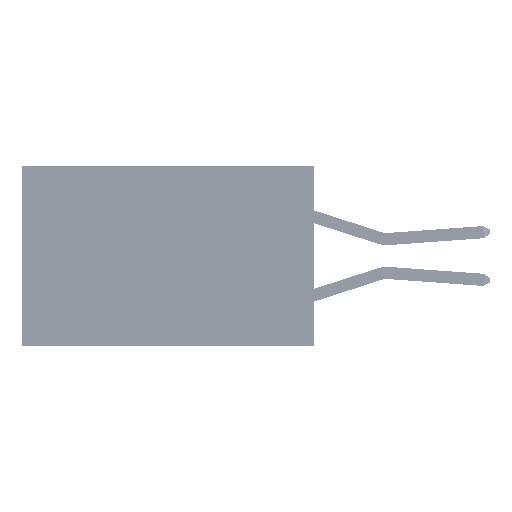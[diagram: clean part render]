
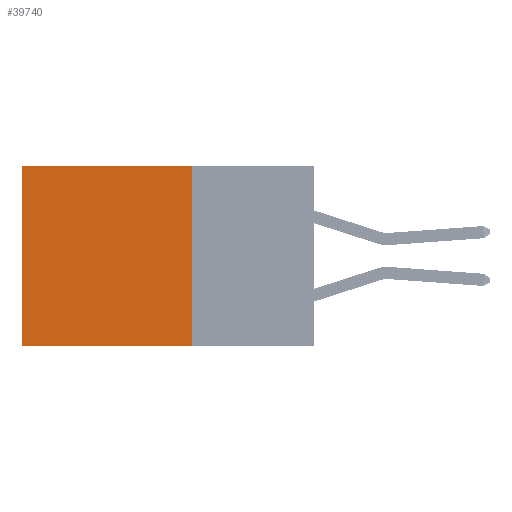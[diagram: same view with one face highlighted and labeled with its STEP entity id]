
A CAD part, left-side view. The second image highlights one B-rep face of the part: STEP entity #39740.
In plain terms, the highlighted planar face has unit normal (-1, 0, 0).
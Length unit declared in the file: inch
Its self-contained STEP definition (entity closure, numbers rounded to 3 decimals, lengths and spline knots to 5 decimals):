
#4793 = LINE ( 'NONE', #19022, #48191 ) ;
#5552 = CARTESIAN_POINT ( 'NONE',  ( 0.2875, 0.25, -0.37 ) ) ;
#8024 = EDGE_CURVE ( 'NONE', #40173, #30002, #37745, .T. ) ;
#10250 = ORIENTED_EDGE ( 'NONE', *, *, #41633, .F. ) ;
#10904 = PLANE ( 'NONE',  #35737 ) ;
#12979 = EDGE_CURVE ( 'NONE', #13496, #30002, #18428, .T. ) ;
#13168 = CARTESIAN_POINT ( 'NONE',  ( 0.2875, 0.6, 0. ) ) ;
#13496 = VERTEX_POINT ( 'NONE', #5552 ) ;
#18175 = FACE_OUTER_BOUND ( 'NONE', #23469, .T. ) ;
#18428 = LINE ( 'NONE', #21665, #22734 ) ;
#18670 = DIRECTION ( 'NONE',  ( 0., 0., -1. ) ) ;
#18850 = DIRECTION ( 'NONE',  ( 0., 1., 0. ) ) ;
#18892 = CARTESIAN_POINT ( 'NONE',  ( 0.2875, 0.25, 0. ) ) ;
#19022 = CARTESIAN_POINT ( 'NONE',  ( 0.2875, 0.25, 0. ) ) ;
#21665 = CARTESIAN_POINT ( 'NONE',  ( 0.2875, 0.25, -0.37 ) ) ;
#21959 = EDGE_CURVE ( 'NONE', #38880, #40173, #43248, .T. ) ;
#22734 = VECTOR ( 'NONE', #29440, 39.37008 ) ;
#23351 = DIRECTION ( 'NONE',  ( 1., 0., 0. ) ) ;
#23430 = VECTOR ( 'NONE', #18850, 39.37008 ) ;
#23469 = EDGE_LOOP ( 'NONE', ( #44778, #27555, #10250, #23684 ) ) ;
#23684 = ORIENTED_EDGE ( 'NONE', *, *, #21959, .T. ) ;
#26060 = CARTESIAN_POINT ( 'NONE',  ( 0.2875, 0.6, 0. ) ) ;
#27555 = ORIENTED_EDGE ( 'NONE', *, *, #12979, .F. ) ;
#29440 = DIRECTION ( 'NONE',  ( 0., 1., 0. ) ) ;
#30002 = VERTEX_POINT ( 'NONE', #44518 ) ;
#31537 = VECTOR ( 'NONE', #48194, 39.37008 ) ;
#35737 = AXIS2_PLACEMENT_3D ( 'NONE', #50528, #23351, #18670 ) ;
#37745 = LINE ( 'NONE', #13168, #31537 ) ;
#38880 = VERTEX_POINT ( 'NONE', #18892 ) ;
#38937 = CARTESIAN_POINT ( 'NONE',  ( 0.2875, 0.25, 0. ) ) ;
#39740 = ADVANCED_FACE ( 'NONE', ( #18175 ), #10904, .F. ) ;
#40173 = VERTEX_POINT ( 'NONE', #26060 ) ;
#41633 = EDGE_CURVE ( 'NONE', #38880, #13496, #4793, .T. ) ;
#43248 = LINE ( 'NONE', #38937, #23430 ) ;
#44518 = CARTESIAN_POINT ( 'NONE',  ( 0.2875, 0.6, -0.37 ) ) ;
#44778 = ORIENTED_EDGE ( 'NONE', *, *, #8024, .T. ) ;
#48191 = VECTOR ( 'NONE', #50195, 39.37008 ) ;
#48194 = DIRECTION ( 'NONE',  ( 0., 0., -1. ) ) ;
#50195 = DIRECTION ( 'NONE',  ( 0., 0., -1. ) ) ;
#50528 = CARTESIAN_POINT ( 'NONE',  ( 0.2875, 0.25, 0. ) ) ;
